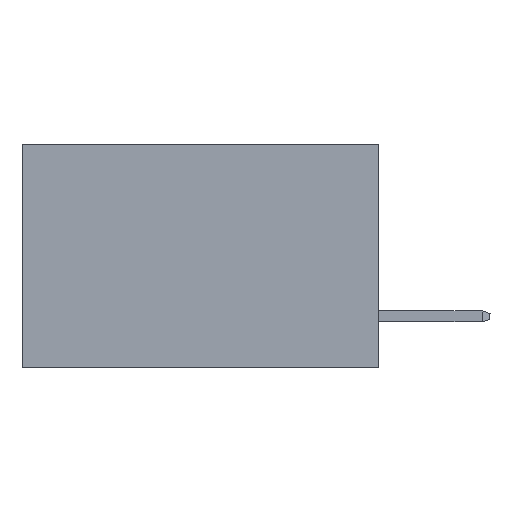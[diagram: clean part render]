
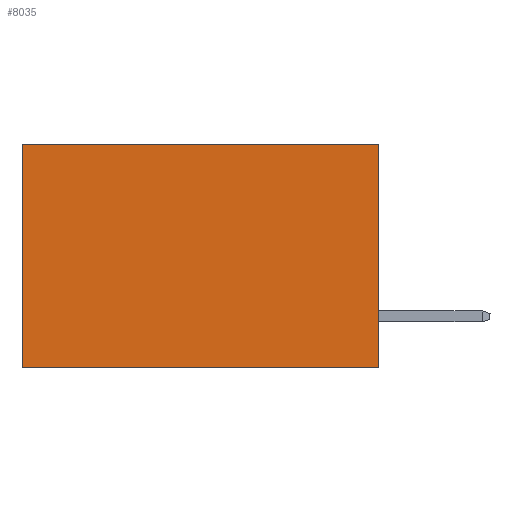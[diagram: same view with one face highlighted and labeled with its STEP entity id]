
A CAD part, left-side view. The second image highlights one B-rep face of the part: STEP entity #8035.
In plain terms, the highlighted planar face has unit normal (-1, 0, 0).
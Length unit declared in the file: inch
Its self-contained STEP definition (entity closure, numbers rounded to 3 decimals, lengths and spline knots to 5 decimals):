
#241 = LINE ( 'NONE', #11240, #7682 ) ;
#322 = CARTESIAN_POINT ( 'NONE',  ( 0.277, 0.59, -0.37 ) ) ;
#1574 = VERTEX_POINT ( 'NONE', #322 ) ;
#1856 = DIRECTION ( 'NONE',  ( 0., 0., -1. ) ) ;
#1966 = DIRECTION ( 'NONE',  ( 1., 0., 0. ) ) ;
#2167 = PLANE ( 'NONE',  #6035 ) ;
#2417 = CARTESIAN_POINT ( 'NONE',  ( 0.277, 0., -0.37 ) ) ;
#2509 = DIRECTION ( 'NONE',  ( 0., 0., -1. ) ) ;
#2680 = ORIENTED_EDGE ( 'NONE', *, *, #6297, .T. ) ;
#2755 = CARTESIAN_POINT ( 'NONE',  ( 0.277, 0., -0.37 ) ) ;
#3563 = LINE ( 'NONE', #2755, #14849 ) ;
#4201 = CARTESIAN_POINT ( 'NONE',  ( 0.277, 0., -0.37 ) ) ;
#4829 = EDGE_CURVE ( 'NONE', #11081, #8406, #9357, .T. ) ;
#5012 = EDGE_LOOP ( 'NONE', ( #2680, #12872, #11709, #17210 ) ) ;
#5647 = EDGE_CURVE ( 'NONE', #10573, #1574, #6600, .T. ) ;
#6035 = AXIS2_PLACEMENT_3D ( 'NONE', #2417, #1966, #1856 ) ;
#6125 = VECTOR ( 'NONE', #18761, 39.37008 ) ;
#6297 = EDGE_CURVE ( 'NONE', #8406, #1574, #241, .T. ) ;
#6600 = LINE ( 'NONE', #19015, #6125 ) ;
#6981 = EDGE_CURVE ( 'NONE', #11081, #10573, #3563, .T. ) ;
#7682 = VECTOR ( 'NONE', #11466, 39.37008 ) ;
#8035 = ADVANCED_FACE ( 'NONE', ( #18401 ), #2167, .F. ) ;
#8213 = CARTESIAN_POINT ( 'NONE',  ( 0.277, 0., 0. ) ) ;
#8214 = DIRECTION ( 'NONE',  ( 0., 1., 0. ) ) ;
#8291 = CARTESIAN_POINT ( 'NONE',  ( 0.277, 0.59, 0. ) ) ;
#8406 = VERTEX_POINT ( 'NONE', #8291 ) ;
#9357 = LINE ( 'NONE', #8213, #16765 ) ;
#10573 = VERTEX_POINT ( 'NONE', #4201 ) ;
#11081 = VERTEX_POINT ( 'NONE', #18157 ) ;
#11240 = CARTESIAN_POINT ( 'NONE',  ( 0.277, 0.59, -0.37 ) ) ;
#11466 = DIRECTION ( 'NONE',  ( 0., 0., -1. ) ) ;
#11709 = ORIENTED_EDGE ( 'NONE', *, *, #6981, .F. ) ;
#12872 = ORIENTED_EDGE ( 'NONE', *, *, #5647, .F. ) ;
#14849 = VECTOR ( 'NONE', #2509, 39.37008 ) ;
#16765 = VECTOR ( 'NONE', #8214, 39.37008 ) ;
#17210 = ORIENTED_EDGE ( 'NONE', *, *, #4829, .T. ) ;
#18157 = CARTESIAN_POINT ( 'NONE',  ( 0.277, 0., 0. ) ) ;
#18401 = FACE_OUTER_BOUND ( 'NONE', #5012, .T. ) ;
#18761 = DIRECTION ( 'NONE',  ( 0., 1., 0. ) ) ;
#19015 = CARTESIAN_POINT ( 'NONE',  ( 0.277, 0., -0.37 ) ) ;
